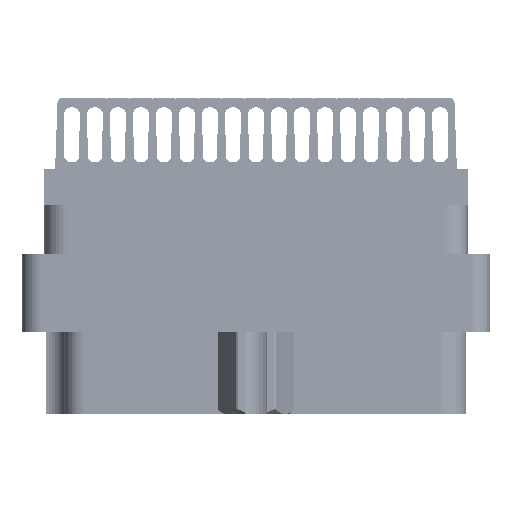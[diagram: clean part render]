
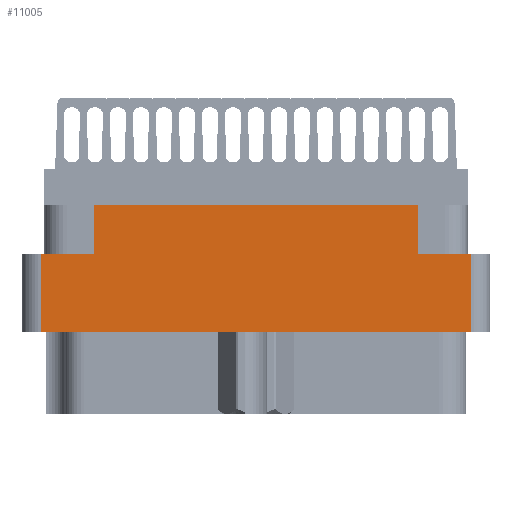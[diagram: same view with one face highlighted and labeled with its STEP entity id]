
A CAD part, left-side view. The second image highlights one B-rep face of the part: STEP entity #11005.
In plain terms, the highlighted planar face has unit normal (-1, 0, 0).
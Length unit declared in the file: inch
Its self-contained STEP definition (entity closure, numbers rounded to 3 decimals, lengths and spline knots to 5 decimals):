
#1353 = EDGE_CURVE ( 'NONE', #82624, #54901, #79654, .T. ) ;
#2483 = CARTESIAN_POINT ( 'NONE',  ( -1.375, -0.5285, -0.277 ) ) ;
#3272 = CARTESIAN_POINT ( 'NONE',  ( -1.375, 0.7005, -0.798 ) ) ;
#4344 = EDGE_CURVE ( 'NONE', #64588, #62866, #84218, .T. ) ;
#5946 = ORIENTED_EDGE ( 'NONE', *, *, #4344, .F. ) ;
#6430 = CARTESIAN_POINT ( 'NONE',  ( -1.375, 0.5285, -0.277 ) ) ;
#6590 = CARTESIAN_POINT ( 'NONE',  ( -1.375, 0., -0.277 ) ) ;
#8625 = VERTEX_POINT ( 'NONE', #90832 ) ;
#9139 = CARTESIAN_POINT ( 'NONE',  ( -1.375, -0.7005, -0.798 ) ) ;
#9399 = CARTESIAN_POINT ( 'NONE',  ( -1.375, -0.5285, -0.117 ) ) ;
#11005 = ADVANCED_FACE ( 'NONE', ( #51658 ), #54278, .T. ) ;
#12127 = VECTOR ( 'NONE', #95494, 39.37008 ) ;
#13499 = VECTOR ( 'NONE', #74686, 39.37008 ) ;
#14339 = VECTOR ( 'NONE', #90150, 39.37008 ) ;
#15347 = CARTESIAN_POINT ( 'NONE',  ( -1.375, 0.7005, -0.277 ) ) ;
#16452 = CARTESIAN_POINT ( 'NONE',  ( -1.375, 0., -0.529 ) ) ;
#17576 = ORIENTED_EDGE ( 'NONE', *, *, #54201, .T. ) ;
#21772 = VECTOR ( 'NONE', #60518, 39.37008 ) ;
#22685 = DIRECTION ( 'NONE',  ( 0., -1., 0. ) ) ;
#24789 = LINE ( 'NONE', #16452, #43652 ) ;
#25608 = DIRECTION ( 'NONE',  ( 0., 0., 1. ) ) ;
#26046 = EDGE_CURVE ( 'NONE', #87895, #54901, #24789, .T. ) ;
#29710 = CARTESIAN_POINT ( 'NONE',  ( -1.375, -0.7625, -0.798 ) ) ;
#30029 = DIRECTION ( 'NONE',  ( -1., 0., 0. ) ) ;
#30994 = CARTESIAN_POINT ( 'NONE',  ( -1.375, 0.5285, -0.277 ) ) ;
#31163 = ORIENTED_EDGE ( 'NONE', *, *, #71254, .F. ) ;
#31593 = ORIENTED_EDGE ( 'NONE', *, *, #98882, .T. ) ;
#35981 = VECTOR ( 'NONE', #22685, 39.37008 ) ;
#37537 = DIRECTION ( 'NONE',  ( 0., -1., 0. ) ) ;
#38796 = VERTEX_POINT ( 'NONE', #102442 ) ;
#40552 = CARTESIAN_POINT ( 'NONE',  ( -1.375, 0.5285, -0.117 ) ) ;
#40663 = DIRECTION ( 'NONE',  ( 0., 1., 0. ) ) ;
#40867 = LINE ( 'NONE', #9139, #61013 ) ;
#43215 = ORIENTED_EDGE ( 'NONE', *, *, #63921, .F. ) ;
#43652 = VECTOR ( 'NONE', #40663, 39.37008 ) ;
#44713 = CARTESIAN_POINT ( 'NONE',  ( -1.375, 0., -0.277 ) ) ;
#50208 = CARTESIAN_POINT ( 'NONE',  ( -1.375, 0.7625, -0.117 ) ) ;
#51658 = FACE_OUTER_BOUND ( 'NONE', #51918, .T. ) ;
#51918 = EDGE_LOOP ( 'NONE', ( #78878, #76346, #55809, #17576, #31163, #31593, #5946, #43215 ) ) ;
#54201 = EDGE_CURVE ( 'NONE', #87895, #38796, #40867, .T. ) ;
#54278 = PLANE ( 'NONE',  #73895 ) ;
#54901 = VERTEX_POINT ( 'NONE', #73220 ) ;
#55809 = ORIENTED_EDGE ( 'NONE', *, *, #26046, .F. ) ;
#60518 = DIRECTION ( 'NONE',  ( 0., -1., 0. ) ) ;
#61013 = VECTOR ( 'NONE', #25608, 39.37008 ) ;
#61962 = DIRECTION ( 'NONE',  ( 0., 0., 1. ) ) ;
#62866 = VERTEX_POINT ( 'NONE', #9399 ) ;
#63921 = EDGE_CURVE ( 'NONE', #68914, #64588, #102441, .T. ) ;
#64588 = VERTEX_POINT ( 'NONE', #40552 ) ;
#68914 = VERTEX_POINT ( 'NONE', #6430 ) ;
#71254 = EDGE_CURVE ( 'NONE', #8625, #38796, #74966, .T. ) ;
#73220 = CARTESIAN_POINT ( 'NONE',  ( -1.375, 0.7005, -0.529 ) ) ;
#73895 = AXIS2_PLACEMENT_3D ( 'NONE', #29710, #30029, #61962 ) ;
#74686 = DIRECTION ( 'NONE',  ( 0., 0., 1. ) ) ;
#74966 = LINE ( 'NONE', #6590, #35981 ) ;
#76346 = ORIENTED_EDGE ( 'NONE', *, *, #1353, .T. ) ;
#78878 = ORIENTED_EDGE ( 'NONE', *, *, #101563, .F. ) ;
#79654 = LINE ( 'NONE', #3272, #14339 ) ;
#82527 = LINE ( 'NONE', #2483, #13499 ) ;
#82624 = VERTEX_POINT ( 'NONE', #15347 ) ;
#84218 = LINE ( 'NONE', #50208, #102980 ) ;
#87895 = VERTEX_POINT ( 'NONE', #98653 ) ;
#90150 = DIRECTION ( 'NONE',  ( 0., 0., -1. ) ) ;
#90832 = CARTESIAN_POINT ( 'NONE',  ( -1.375, -0.5285, -0.277 ) ) ;
#95494 = DIRECTION ( 'NONE',  ( 0., 0., 1. ) ) ;
#98653 = CARTESIAN_POINT ( 'NONE',  ( -1.375, -0.7005, -0.529 ) ) ;
#98882 = EDGE_CURVE ( 'NONE', #8625, #62866, #82527, .T. ) ;
#100844 = LINE ( 'NONE', #44713, #21772 ) ;
#101563 = EDGE_CURVE ( 'NONE', #82624, #68914, #100844, .T. ) ;
#102441 = LINE ( 'NONE', #30994, #12127 ) ;
#102442 = CARTESIAN_POINT ( 'NONE',  ( -1.375, -0.7005, -0.277 ) ) ;
#102980 = VECTOR ( 'NONE', #37537, 39.37008 ) ;
